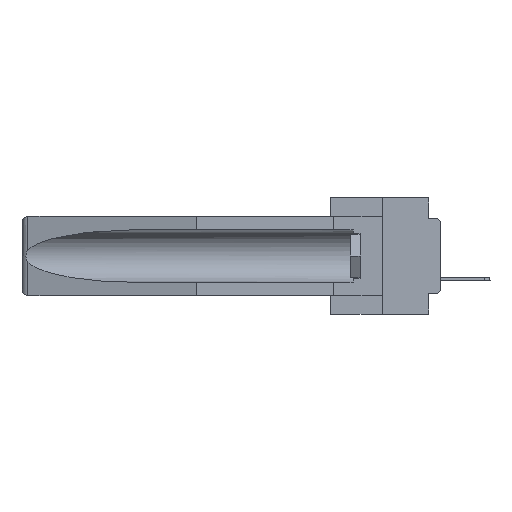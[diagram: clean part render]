
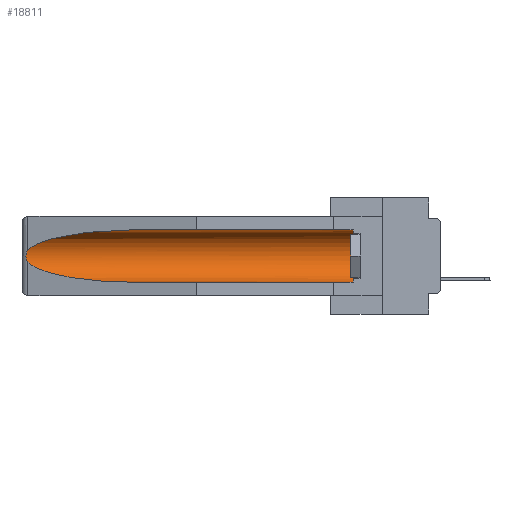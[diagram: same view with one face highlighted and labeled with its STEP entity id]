
A CAD part, left-side view. The second image highlights one B-rep face of the part: STEP entity #18811.
In plain terms, the highlighted cylindrical face has radius 2.857 mm (diameter 5.715 mm), a partial arc.
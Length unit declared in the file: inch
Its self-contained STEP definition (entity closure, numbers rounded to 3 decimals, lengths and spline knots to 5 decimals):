
#2 = DIRECTION ( 'NONE',  ( 0., 0., 1. ) ) ;
#491 = EDGE_CURVE ( 'NONE', #23196, #7315, #23453, .T. ) ;
#1052 = CARTESIAN_POINT ( 'NONE',  ( 0.155, 0.126, -0.284 ) ) ;
#1427 = DIRECTION ( 'NONE',  ( 0., 1., 0. ) ) ;
#1487 = CARTESIAN_POINT ( 'NONE',  ( 0.155, 0.126, -0.059 ) ) ;
#1804 = VERTEX_POINT ( 'NONE', #1052 ) ;
#1846 = VERTEX_POINT ( 'NONE', #29616 ) ;
#2304 = CARTESIAN_POINT ( 'NONE',  ( 0.21114, 1.30732, -0.059 ) ) ;
#2330 = CARTESIAN_POINT ( 'NONE',  ( 0.2675, 1.53308, -0.17534 ) ) ;
#3512 = ORIENTED_EDGE ( 'NONE', *, *, #491, .T. ) ;
#4268 = EDGE_CURVE ( 'NONE', #6279, #23196, #21411, .T. ) ;
#6279 = VERTEX_POINT ( 'NONE', #18593 ) ;
#6369 = CARTESIAN_POINT ( 'NONE',  ( 0.26537, 1.52718, -0.14972 ) ) ;
#7315 = VERTEX_POINT ( 'NONE', #7789 ) ;
#7789 = CARTESIAN_POINT ( 'NONE',  ( 0.155, 1.07973, -0.284 ) ) ;
#8498 = LINE ( 'NONE', #11261, #9758 ) ;
#8632 = ORIENTED_EDGE ( 'NONE', *, *, #11549, .T. ) ;
#8741 = AXIS2_PLACEMENT_3D ( 'NONE', #10364, #27870, #2 ) ;
#8842 = DIRECTION ( 'NONE',  ( 0., 0., 1. ) ) ;
#9758 = VECTOR ( 'NONE', #26494, 39.37008 ) ;
#9820 = CARTESIAN_POINT ( 'NONE',  ( 0.26537, 1.52718, -0.14972 ) ) ;
#10023 = CARTESIAN_POINT ( 'NONE',  ( 0.2673, 1.5327, -0.16383 ) ) ;
#10303 = ORIENTED_EDGE ( 'NONE', *, *, #19488, .F. ) ;
#10364 = CARTESIAN_POINT ( 'NONE',  ( 0.155, 0.126, -0.1715 ) ) ;
#10801 = CARTESIAN_POINT ( 'NONE',  ( 0.21114, 1.30732, -0.284 ) ) ;
#11261 = CARTESIAN_POINT ( 'NONE',  ( 0.155, -0.30754, -0.059 ) ) ;
#11549 = EDGE_CURVE ( 'NONE', #1804, #14424, #17945, .T. ) ;
#11752 = DIRECTION ( 'NONE',  ( 0., 1., 0. ) ) ;
#12708 = CARTESIAN_POINT ( 'NONE',  ( 0.26537, 1.52718, -0.19328 ) ) ;
#12886 = CYLINDRICAL_SURFACE ( 'NONE', #18354, 0.1125 ) ;
#14424 = VERTEX_POINT ( 'NONE', #1487 ) ;
#15318 = CARTESIAN_POINT ( 'NONE',  ( 0.26597, 1.5296, -0.19026 ) ) ;
#15326 = FACE_OUTER_BOUND ( 'NONE', #29902, .T. ) ;
#15681 = CARTESIAN_POINT ( 'NONE',  ( 0.155, 1.07973, -0.284 ) ) ;
#16313 = EDGE_CURVE ( 'NONE', #1846, #6279, #18965, .T. ) ;
#16595 = CARTESIAN_POINT ( 'NONE',  ( 0.25451, 1.48313, -0.09465 ) ) ;
#16698 = CARTESIAN_POINT ( 'NONE',  ( 0.155, -0.30754, -0.1715 ) ) ;
#17755 = CARTESIAN_POINT ( 'NONE',  ( 0.26654, 1.53092, -0.15636 ) ) ;
#17945 = CIRCLE ( 'NONE', #8741, 0.1125 ) ;
#18354 = AXIS2_PLACEMENT_3D ( 'NONE', #16698, #11752, #8842 ) ;
#18593 = CARTESIAN_POINT ( 'NONE',  ( 0.26537, 1.52718, -0.14972 ) ) ;
#18811 = ADVANCED_FACE ( 'NONE', ( #15326 ), #12886, .F. ) ;
#18965 =( BOUNDED_CURVE ( )  B_SPLINE_CURVE ( 3, ( #33101, #2304, #16595, #6369 ),
 .UNSPECIFIED., .F., .F. ) 
 B_SPLINE_CURVE_WITH_KNOTS ( ( 4, 4 ),
 ( 4.71239, 6.08839 ),
 .UNSPECIFIED. ) 
 CURVE ( )  GEOMETRIC_REPRESENTATION_ITEM ( )  RATIONAL_B_SPLINE_CURVE ( ( 1., 0.848, 0.848, 1. ) ) 
 REPRESENTATION_ITEM ( '' )  );
#19488 = EDGE_CURVE ( 'NONE', #1804, #7315, #19634, .T. ) ;
#19634 = LINE ( 'NONE', #32202, #22851 ) ;
#20330 = ORIENTED_EDGE ( 'NONE', *, *, #16313, .T. ) ;
#20422 = CARTESIAN_POINT ( 'NONE',  ( 0.26597, 1.52961, -0.15275 ) ) ;
#21411 = B_SPLINE_CURVE_WITH_KNOTS ( 'NONE', 3,
 ( #9820, #20422, #17755, #10023, #32902, #2330, #25475, #30425, #15318, #12708 ),
 .UNSPECIFIED., .F., .F.,
 ( 4, 2, 2, 2, 4 ),
 ( 0., 0.00029, 0.00058, 0.00087, 0.00117 ),
 .UNSPECIFIED. ) ;
#21563 = ORIENTED_EDGE ( 'NONE', *, *, #22223, .T. ) ;
#22223 = EDGE_CURVE ( 'NONE', #14424, #1846, #8498, .T. ) ;
#22851 = VECTOR ( 'NONE', #1427, 39.37008 ) ;
#23196 = VERTEX_POINT ( 'NONE', #24590 ) ;
#23453 =( BOUNDED_CURVE ( )  B_SPLINE_CURVE ( 3, ( #25850, #26050, #10801, #15681 ),
 .UNSPECIFIED., .F., .F. ) 
 B_SPLINE_CURVE_WITH_KNOTS ( ( 4, 4 ),
 ( 0.1948, 1.5708 ),
 .UNSPECIFIED. ) 
 CURVE ( )  GEOMETRIC_REPRESENTATION_ITEM ( )  RATIONAL_B_SPLINE_CURVE ( ( 1., 0.848, 0.848, 1. ) ) 
 REPRESENTATION_ITEM ( '' )  );
#24590 = CARTESIAN_POINT ( 'NONE',  ( 0.26537, 1.52718, -0.19328 ) ) ;
#25475 = CARTESIAN_POINT ( 'NONE',  ( 0.2673, 1.53269, -0.17917 ) ) ;
#25850 = CARTESIAN_POINT ( 'NONE',  ( 0.26537, 1.52718, -0.19328 ) ) ;
#26050 = CARTESIAN_POINT ( 'NONE',  ( 0.25451, 1.48313, -0.24835 ) ) ;
#26494 = DIRECTION ( 'NONE',  ( 0., 1., 0. ) ) ;
#27870 = DIRECTION ( 'NONE',  ( 0., -1., 0. ) ) ;
#29616 = CARTESIAN_POINT ( 'NONE',  ( 0.155, 1.07973, -0.059 ) ) ;
#29902 = EDGE_LOOP ( 'NONE', ( #20330, #31596, #3512, #10303, #8632, #21563 ) ) ;
#30425 = CARTESIAN_POINT ( 'NONE',  ( 0.26655, 1.53094, -0.18657 ) ) ;
#31596 = ORIENTED_EDGE ( 'NONE', *, *, #4268, .T. ) ;
#32202 = CARTESIAN_POINT ( 'NONE',  ( 0.155, -0.30754, -0.284 ) ) ;
#32902 = CARTESIAN_POINT ( 'NONE',  ( 0.2675, 1.53308, -0.16763 ) ) ;
#33101 = CARTESIAN_POINT ( 'NONE',  ( 0.155, 1.07973, -0.059 ) ) ;
